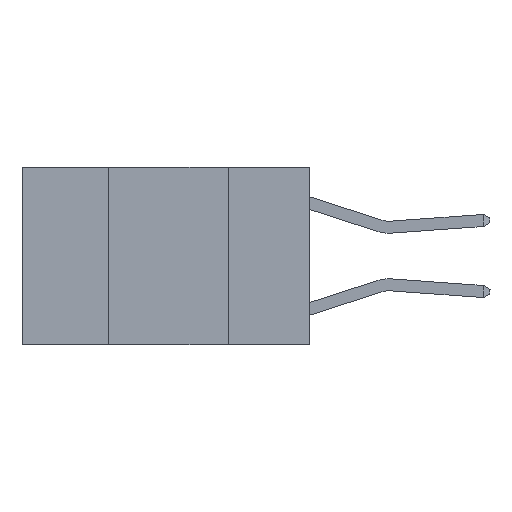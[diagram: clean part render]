
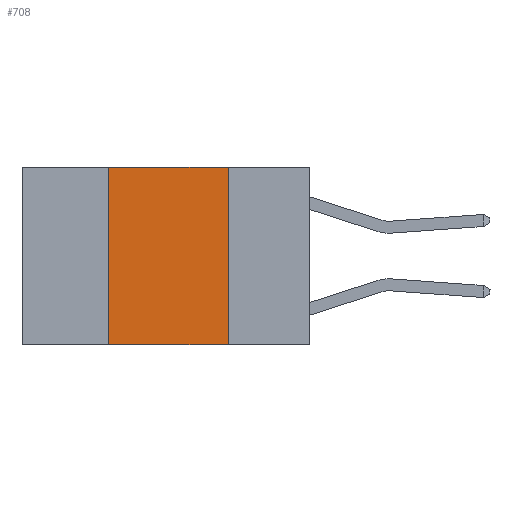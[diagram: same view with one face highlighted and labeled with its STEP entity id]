
A CAD part, left-side view. The second image highlights one B-rep face of the part: STEP entity #708.
In plain terms, the highlighted planar face has unit normal (-1, 0, 0).
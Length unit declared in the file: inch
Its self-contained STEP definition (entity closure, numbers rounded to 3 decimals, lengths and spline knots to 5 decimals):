
#71 = ORIENTED_EDGE ( 'NONE', *, *, #8360, .T. ) ;
#415 = CARTESIAN_POINT ( 'NONE',  ( 0., 0.17, -0.37 ) ) ;
#519 = DIRECTION ( 'NONE',  ( 0., 0., 1. ) ) ;
#708 = ADVANCED_FACE ( 'NONE', ( #3664 ), #1848, .F. ) ;
#1082 = DIRECTION ( 'NONE',  ( 1., 0., 0. ) ) ;
#1209 = CARTESIAN_POINT ( 'NONE',  ( 0., 0.6, 0. ) ) ;
#1211 = ORIENTED_EDGE ( 'NONE', *, *, #7528, .F. ) ;
#1406 = CARTESIAN_POINT ( 'NONE',  ( 0., 0.42, -0.37 ) ) ;
#1601 = VERTEX_POINT ( 'NONE', #5777 ) ;
#1848 = PLANE ( 'NONE',  #7366 ) ;
#1850 = VECTOR ( 'NONE', #519, 39.37008 ) ;
#1989 = LINE ( 'NONE', #7110, #1850 ) ;
#2198 = CARTESIAN_POINT ( 'NONE',  ( 0., 0.42, 0. ) ) ;
#2583 = VERTEX_POINT ( 'NONE', #1406 ) ;
#2757 = VECTOR ( 'NONE', #3739, 39.37008 ) ;
#2941 = EDGE_LOOP ( 'NONE', ( #1211, #5637, #3688, #71 ) ) ;
#3214 = CARTESIAN_POINT ( 'NONE',  ( 0., 0.6, -0.37 ) ) ;
#3503 = VECTOR ( 'NONE', #5893, 39.37008 ) ;
#3664 = FACE_OUTER_BOUND ( 'NONE', #2941, .T. ) ;
#3688 = ORIENTED_EDGE ( 'NONE', *, *, #7432, .F. ) ;
#3710 = EDGE_CURVE ( 'NONE', #7666, #1601, #5160, .T. ) ;
#3739 = DIRECTION ( 'NONE',  ( 0., -1., 0. ) ) ;
#4412 = DIRECTION ( 'NONE',  ( 0., 0., -1. ) ) ;
#5160 = LINE ( 'NONE', #6506, #2757 ) ;
#5637 = ORIENTED_EDGE ( 'NONE', *, *, #3710, .F. ) ;
#5777 = CARTESIAN_POINT ( 'NONE',  ( 0., 0.17, 0. ) ) ;
#5893 = DIRECTION ( 'NONE',  ( 0., -1., 0. ) ) ;
#6404 = VECTOR ( 'NONE', #8516, 39.37008 ) ;
#6506 = CARTESIAN_POINT ( 'NONE',  ( 0., 0.6, 0. ) ) ;
#7110 = CARTESIAN_POINT ( 'NONE',  ( 0., 0.42, 0. ) ) ;
#7366 = AXIS2_PLACEMENT_3D ( 'NONE', #1209, #1082, #4412 ) ;
#7432 = EDGE_CURVE ( 'NONE', #2583, #7666, #1989, .T. ) ;
#7528 = EDGE_CURVE ( 'NONE', #1601, #8131, #7800, .T. ) ;
#7666 = VERTEX_POINT ( 'NONE', #2198 ) ;
#7800 = LINE ( 'NONE', #7841, #6404 ) ;
#7841 = CARTESIAN_POINT ( 'NONE',  ( 0., 0.17, 0. ) ) ;
#7857 = LINE ( 'NONE', #3214, #3503 ) ;
#8131 = VERTEX_POINT ( 'NONE', #415 ) ;
#8360 = EDGE_CURVE ( 'NONE', #2583, #8131, #7857, .T. ) ;
#8516 = DIRECTION ( 'NONE',  ( 0., 0., -1. ) ) ;
